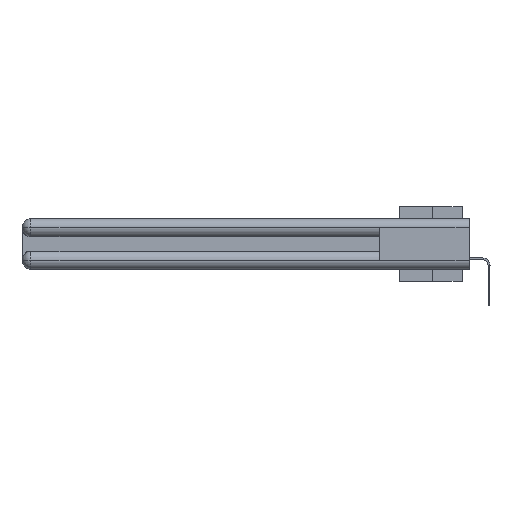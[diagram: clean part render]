
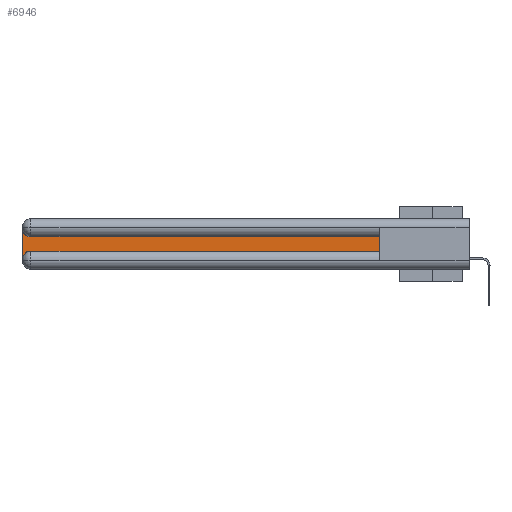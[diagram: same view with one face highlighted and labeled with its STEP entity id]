
A CAD part, left-side view. The second image highlights one B-rep face of the part: STEP entity #6946.
In plain terms, the highlighted planar face has unit normal (-1, 0, 0).
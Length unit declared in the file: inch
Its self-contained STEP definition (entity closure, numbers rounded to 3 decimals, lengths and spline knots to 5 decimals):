
#179 = DIRECTION ( 'NONE',  ( 0., 1., 0. ) ) ;
#422 = ORIENTED_EDGE ( 'NONE', *, *, #30521, .T. ) ;
#635 = DIRECTION ( 'NONE',  ( 0., -1., 0. ) ) ;
#642 = VERTEX_POINT ( 'NONE', #4124 ) ;
#1101 = CARTESIAN_POINT ( 'NONE',  ( 0.075, 3., -0.0625 ) ) ;
#2823 = EDGE_CURVE ( 'NONE', #17107, #19532, #23161, .T. ) ;
#3435 = VERTEX_POINT ( 'NONE', #1101 ) ;
#4124 = CARTESIAN_POINT ( 'NONE',  ( 0.075, 3., -0.2775 ) ) ;
#4715 = LINE ( 'NONE', #40205, #30423 ) ;
#6217 = DIRECTION ( 'NONE',  ( 0., 0., -1. ) ) ;
#6783 = DIRECTION ( 'NONE',  ( 0., 0., -1. ) ) ;
#6946 = ADVANCED_FACE ( 'NONE', ( #28482 ), #30890, .F. ) ;
#8512 = CIRCLE ( 'NONE', #25407, 0.06 ) ;
#9029 = VECTOR ( 'NONE', #33669, 39.37008 ) ;
#12263 = DIRECTION ( 'NONE',  ( 0., 0., -1. ) ) ;
#12316 = DIRECTION ( 'NONE',  ( 1., 0., 0. ) ) ;
#12362 = CARTESIAN_POINT ( 'NONE',  ( 0.075, 0.6, -0.2175 ) ) ;
#12579 = CIRCLE ( 'NONE', #13525, 0.06 ) ;
#12613 = ORIENTED_EDGE ( 'NONE', *, *, #16892, .T. ) ;
#12781 = CARTESIAN_POINT ( 'NONE',  ( 0.075, 2.94, -0.2175 ) ) ;
#13525 = AXIS2_PLACEMENT_3D ( 'NONE', #38094, #22696, #6783 ) ;
#15448 = CARTESIAN_POINT ( 'NONE',  ( 0.075, 3., -0.1225 ) ) ;
#15657 = EDGE_CURVE ( 'NONE', #642, #36161, #8512, .T. ) ;
#16892 = EDGE_CURVE ( 'NONE', #36161, #17107, #34195, .T. ) ;
#17107 = VERTEX_POINT ( 'NONE', #35231 ) ;
#17540 = EDGE_CURVE ( 'NONE', #19532, #27286, #4715, .T. ) ;
#18378 = CARTESIAN_POINT ( 'NONE',  ( 0.075, 2.94, -0.1225 ) ) ;
#18649 = CARTESIAN_POINT ( 'NONE',  ( 0.075, 0.6, -0.1225 ) ) ;
#19532 = VERTEX_POINT ( 'NONE', #18649 ) ;
#19654 = CARTESIAN_POINT ( 'NONE',  ( 0.075, 0.6, -0.2175 ) ) ;
#21003 = ORIENTED_EDGE ( 'NONE', *, *, #29661, .T. ) ;
#21259 = CARTESIAN_POINT ( 'NONE',  ( 0.075, 3., -0.2175 ) ) ;
#21530 = CARTESIAN_POINT ( 'NONE',  ( 0.075, 2.94, -0.2775 ) ) ;
#22210 = LINE ( 'NONE', #21259, #24155 ) ;
#22696 = DIRECTION ( 'NONE',  ( 1., 0., 0. ) ) ;
#23161 = LINE ( 'NONE', #12362, #9029 ) ;
#24155 = VECTOR ( 'NONE', #33719, 39.37008 ) ;
#24281 = ORIENTED_EDGE ( 'NONE', *, *, #17540, .T. ) ;
#25407 = AXIS2_PLACEMENT_3D ( 'NONE', #21530, #27882, #12263 ) ;
#26588 = ORIENTED_EDGE ( 'NONE', *, *, #2823, .T. ) ;
#27286 = VERTEX_POINT ( 'NONE', #18378 ) ;
#27882 = DIRECTION ( 'NONE',  ( 1., 0., 0. ) ) ;
#28482 = FACE_OUTER_BOUND ( 'NONE', #33368, .T. ) ;
#29306 = VECTOR ( 'NONE', #635, 39.37008 ) ;
#29661 = EDGE_CURVE ( 'NONE', #3435, #642, #22210, .T. ) ;
#30423 = VECTOR ( 'NONE', #179, 39.37008 ) ;
#30521 = EDGE_CURVE ( 'NONE', #27286, #3435, #12579, .T. ) ;
#30545 = AXIS2_PLACEMENT_3D ( 'NONE', #15448, #12316, #6217 ) ;
#30890 = PLANE ( 'NONE',  #30545 ) ;
#33368 = EDGE_LOOP ( 'NONE', ( #24281, #422, #21003, #35994, #12613, #26588 ) ) ;
#33669 = DIRECTION ( 'NONE',  ( 0., 0., 1. ) ) ;
#33719 = DIRECTION ( 'NONE',  ( 0., 0., -1. ) ) ;
#34195 = LINE ( 'NONE', #19654, #29306 ) ;
#35231 = CARTESIAN_POINT ( 'NONE',  ( 0.075, 0.6, -0.2175 ) ) ;
#35994 = ORIENTED_EDGE ( 'NONE', *, *, #15657, .T. ) ;
#36161 = VERTEX_POINT ( 'NONE', #12781 ) ;
#38094 = CARTESIAN_POINT ( 'NONE',  ( 0.075, 2.94, -0.0625 ) ) ;
#40205 = CARTESIAN_POINT ( 'NONE',  ( 0.075, 0.6, -0.1225 ) ) ;
